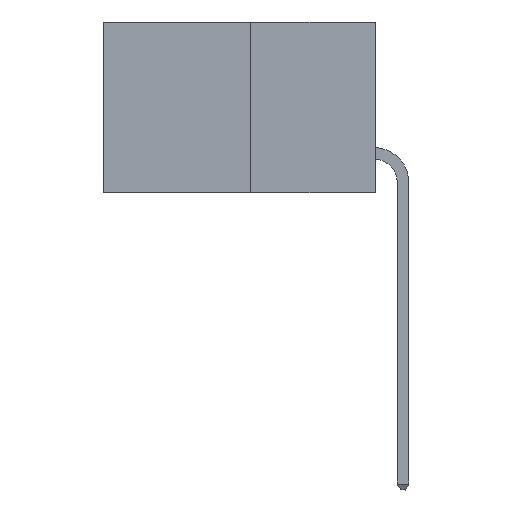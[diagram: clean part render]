
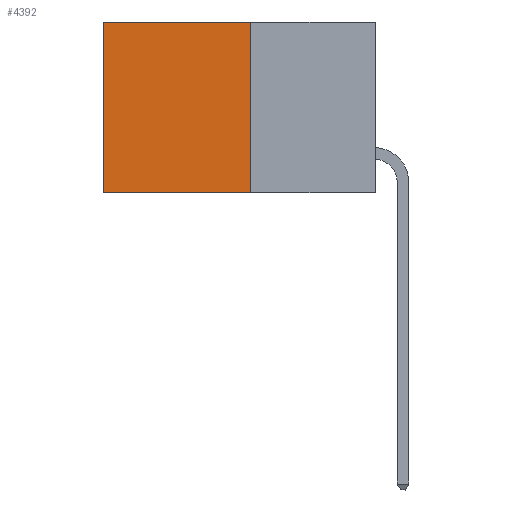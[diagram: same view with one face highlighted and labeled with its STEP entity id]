
A CAD part, left-side view. The second image highlights one B-rep face of the part: STEP entity #4392.
In plain terms, the highlighted planar face has unit normal (-1, 0, 0).
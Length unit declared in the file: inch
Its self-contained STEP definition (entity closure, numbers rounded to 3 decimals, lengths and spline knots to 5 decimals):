
#436 = VECTOR ( 'NONE', #6787, 39.37008 ) ;
#488 = CARTESIAN_POINT ( 'NONE',  ( 0.277, 0.59, -0.37 ) ) ;
#755 = EDGE_CURVE ( 'NONE', #19758, #8555, #21433, .T. ) ;
#965 = ORIENTED_EDGE ( 'NONE', *, *, #1088, .T. ) ;
#1088 = EDGE_CURVE ( 'NONE', #18415, #8555, #12248, .T. ) ;
#2125 = ORIENTED_EDGE ( 'NONE', *, *, #12722, .T. ) ;
#3590 = CARTESIAN_POINT ( 'NONE',  ( 0.277, 0.59, 0. ) ) ;
#4141 = CARTESIAN_POINT ( 'NONE',  ( 0.277, 0.27, -0.37 ) ) ;
#4168 = DIRECTION ( 'NONE',  ( 1., 0., 0. ) ) ;
#4392 = ADVANCED_FACE ( 'NONE', ( #9808 ), #5028, .F. ) ;
#5028 = PLANE ( 'NONE',  #25040 ) ;
#5283 = EDGE_CURVE ( 'NONE', #13017, #19758, #19619, .T. ) ;
#6600 = VECTOR ( 'NONE', #21605, 39.37008 ) ;
#6787 = DIRECTION ( 'NONE',  ( 0., 1., 0. ) ) ;
#7383 = DIRECTION ( 'NONE',  ( 0., 0., -1. ) ) ;
#7417 = CARTESIAN_POINT ( 'NONE',  ( 0.277, 0.27, -0.37 ) ) ;
#8555 = VERTEX_POINT ( 'NONE', #26763 ) ;
#9808 = FACE_OUTER_BOUND ( 'NONE', #13043, .T. ) ;
#10356 = DIRECTION ( 'NONE',  ( 0., 0., -1. ) ) ;
#12248 = LINE ( 'NONE', #488, #6600 ) ;
#12461 = LINE ( 'NONE', #17293, #436 ) ;
#12722 = EDGE_CURVE ( 'NONE', #13017, #18415, #12461, .T. ) ;
#13017 = VERTEX_POINT ( 'NONE', #20304 ) ;
#13043 = EDGE_LOOP ( 'NONE', ( #965, #26121, #15167, #2125 ) ) ;
#14691 = VECTOR ( 'NONE', #7383, 39.37008 ) ;
#15167 = ORIENTED_EDGE ( 'NONE', *, *, #5283, .F. ) ;
#15875 = VECTOR ( 'NONE', #17436, 39.37008 ) ;
#17293 = CARTESIAN_POINT ( 'NONE',  ( 0.277, 0.27, 0. ) ) ;
#17436 = DIRECTION ( 'NONE',  ( 0., 1., 0. ) ) ;
#18415 = VERTEX_POINT ( 'NONE', #3590 ) ;
#19619 = LINE ( 'NONE', #7417, #14691 ) ;
#19758 = VERTEX_POINT ( 'NONE', #24449 ) ;
#20304 = CARTESIAN_POINT ( 'NONE',  ( 0.277, 0.27, 0. ) ) ;
#21433 = LINE ( 'NONE', #21917, #15875 ) ;
#21605 = DIRECTION ( 'NONE',  ( 0., 0., -1. ) ) ;
#21917 = CARTESIAN_POINT ( 'NONE',  ( 0.277, 0.27, -0.37 ) ) ;
#24449 = CARTESIAN_POINT ( 'NONE',  ( 0.277, 0.27, -0.37 ) ) ;
#25040 = AXIS2_PLACEMENT_3D ( 'NONE', #4141, #4168, #10356 ) ;
#26121 = ORIENTED_EDGE ( 'NONE', *, *, #755, .F. ) ;
#26763 = CARTESIAN_POINT ( 'NONE',  ( 0.277, 0.59, -0.37 ) ) ;
